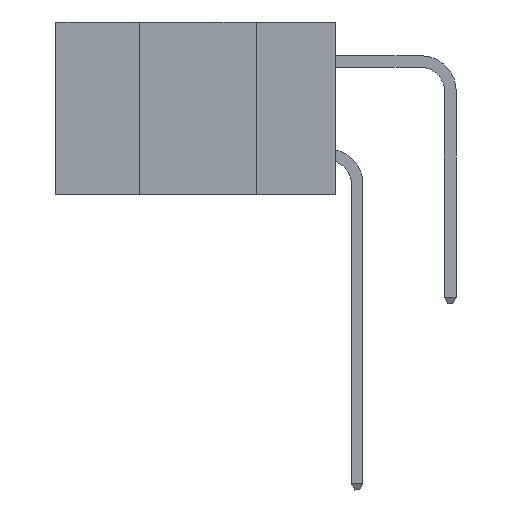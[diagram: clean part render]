
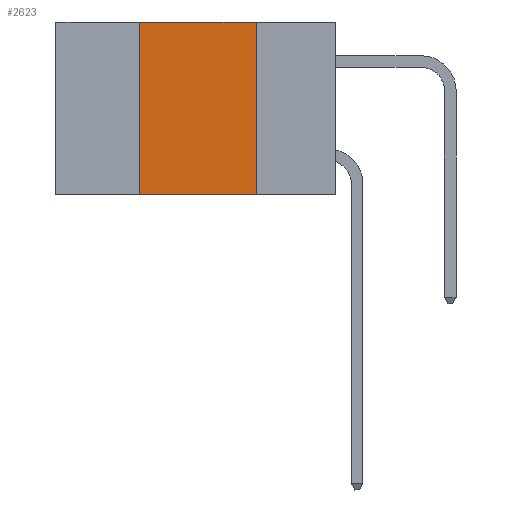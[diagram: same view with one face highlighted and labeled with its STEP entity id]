
A CAD part, left-side view. The second image highlights one B-rep face of the part: STEP entity #2623.
In plain terms, the highlighted planar face has unit normal (-1, 0, 0).
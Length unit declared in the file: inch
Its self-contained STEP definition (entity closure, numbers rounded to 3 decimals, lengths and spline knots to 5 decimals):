
#774 = DIRECTION ( 'NONE',  ( 1., 0., 0. ) ) ;
#1010 = CARTESIAN_POINT ( 'NONE',  ( 0., 0.6, 0. ) ) ;
#1349 = CARTESIAN_POINT ( 'NONE',  ( 0., 0.17, 0. ) ) ;
#1540 = CARTESIAN_POINT ( 'NONE',  ( 0., 0.42, 0. ) ) ;
#1887 = CARTESIAN_POINT ( 'NONE',  ( 0., 0.17, -0.37 ) ) ;
#2084 = VERTEX_POINT ( 'NONE', #17646 ) ;
#2133 = VECTOR ( 'NONE', #25082, 39.37008 ) ;
#2623 = ADVANCED_FACE ( 'NONE', ( #7104 ), #18745, .F. ) ;
#3073 = ORIENTED_EDGE ( 'NONE', *, *, #3163, .T. ) ;
#3163 = EDGE_CURVE ( 'NONE', #5630, #13259, #23243, .T. ) ;
#4222 = EDGE_LOOP ( 'NONE', ( #22662, #25969, #14487, #3073 ) ) ;
#5630 = VERTEX_POINT ( 'NONE', #21553 ) ;
#6173 = VECTOR ( 'NONE', #21265, 39.37008 ) ;
#6682 = LINE ( 'NONE', #1540, #22254 ) ;
#7104 = FACE_OUTER_BOUND ( 'NONE', #4222, .T. ) ;
#8692 = DIRECTION ( 'NONE',  ( 0., 0., -1. ) ) ;
#11914 = CARTESIAN_POINT ( 'NONE',  ( 0., 0.17, 0. ) ) ;
#13259 = VERTEX_POINT ( 'NONE', #1887 ) ;
#14487 = ORIENTED_EDGE ( 'NONE', *, *, #17167, .F. ) ;
#16642 = VECTOR ( 'NONE', #20830, 39.37008 ) ;
#17167 = EDGE_CURVE ( 'NONE', #5630, #2084, #6682, .T. ) ;
#17646 = CARTESIAN_POINT ( 'NONE',  ( 0., 0.42, 0. ) ) ;
#18074 = LINE ( 'NONE', #1349, #2133 ) ;
#18469 = CARTESIAN_POINT ( 'NONE',  ( 0., 0.6, -0.37 ) ) ;
#18717 = EDGE_CURVE ( 'NONE', #20294, #13259, #18074, .T. ) ;
#18745 = PLANE ( 'NONE',  #20936 ) ;
#20294 = VERTEX_POINT ( 'NONE', #11914 ) ;
#20463 = LINE ( 'NONE', #1010, #6173 ) ;
#20830 = DIRECTION ( 'NONE',  ( 0., -1., 0. ) ) ;
#20936 = AXIS2_PLACEMENT_3D ( 'NONE', #25095, #774, #8692 ) ;
#21265 = DIRECTION ( 'NONE',  ( 0., -1., 0. ) ) ;
#21553 = CARTESIAN_POINT ( 'NONE',  ( 0., 0.42, -0.37 ) ) ;
#22254 = VECTOR ( 'NONE', #23883, 39.37008 ) ;
#22662 = ORIENTED_EDGE ( 'NONE', *, *, #18717, .F. ) ;
#23243 = LINE ( 'NONE', #18469, #16642 ) ;
#23883 = DIRECTION ( 'NONE',  ( 0., 0., 1. ) ) ;
#25082 = DIRECTION ( 'NONE',  ( 0., 0., -1. ) ) ;
#25095 = CARTESIAN_POINT ( 'NONE',  ( 0., 0.6, 0. ) ) ;
#25781 = EDGE_CURVE ( 'NONE', #2084, #20294, #20463, .T. ) ;
#25969 = ORIENTED_EDGE ( 'NONE', *, *, #25781, .F. ) ;
